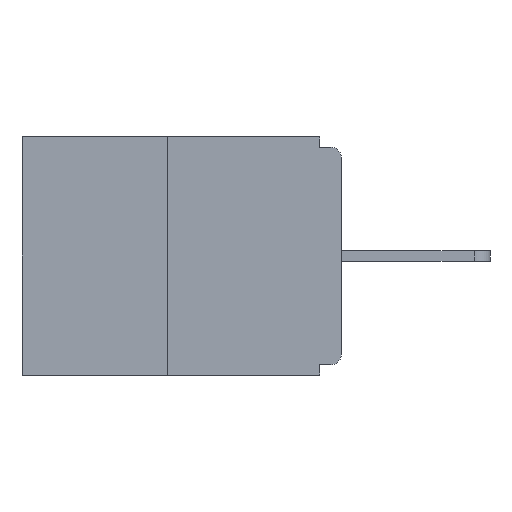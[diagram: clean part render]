
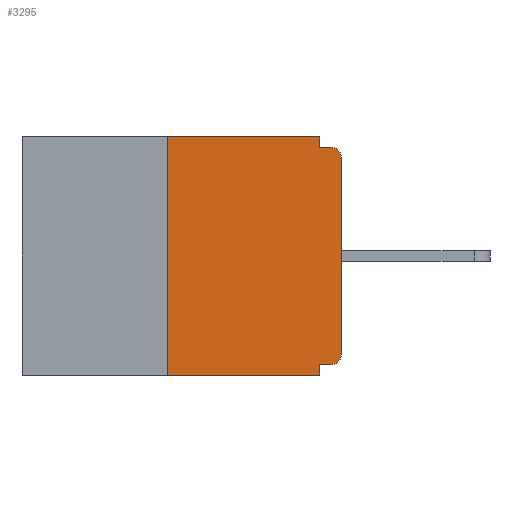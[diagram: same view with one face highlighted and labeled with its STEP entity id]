
A CAD part, left-side view. The second image highlights one B-rep face of the part: STEP entity #3295.
In plain terms, the highlighted planar face has unit normal (-1, 0, 0).
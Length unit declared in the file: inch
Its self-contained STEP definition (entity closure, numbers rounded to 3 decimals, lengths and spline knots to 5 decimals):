
#161 = VECTOR ( 'NONE', #1043, 39.37008 ) ;
#239 = DIRECTION ( 'NONE',  ( 0., 0., -1. ) ) ;
#423 = EDGE_CURVE ( 'NONE', #15129, #9953, #10699, .T. ) ;
#1043 = DIRECTION ( 'NONE',  ( 0., 0., -1. ) ) ;
#1128 = VERTEX_POINT ( 'NONE', #9531 ) ;
#1290 = VECTOR ( 'NONE', #1353, 39.37008 ) ;
#1353 = DIRECTION ( 'NONE',  ( 0., -1., 0. ) ) ;
#1645 = LINE ( 'NONE', #8668, #11271 ) ;
#2139 = EDGE_CURVE ( 'NONE', #6346, #11528, #9240, .T. ) ;
#2276 = ORIENTED_EDGE ( 'NONE', *, *, #6150, .F. ) ;
#3017 = EDGE_CURVE ( 'NONE', #9953, #8100, #14920, .T. ) ;
#3056 = CARTESIAN_POINT ( 'NONE',  ( 0., 0.015, -0.328 ) ) ;
#3295 = ADVANCED_FACE ( 'NONE', ( #3906 ), #15414, .F. ) ;
#3436 = VECTOR ( 'NONE', #5812, 39.37008 ) ;
#3559 = ORIENTED_EDGE ( 'NONE', *, *, #3017, .F. ) ;
#3906 = FACE_OUTER_BOUND ( 'NONE', #9827, .T. ) ;
#4535 = VECTOR ( 'NONE', #5402, 39.37008 ) ;
#4733 = EDGE_CURVE ( 'NONE', #5735, #5807, #5259, .T. ) ;
#4898 = DIRECTION ( 'NONE',  ( -1., 0., 0. ) ) ;
#5259 = LINE ( 'NONE', #17014, #1290 ) ;
#5402 = DIRECTION ( 'NONE',  ( 0., -1., 0. ) ) ;
#5409 = AXIS2_PLACEMENT_3D ( 'NONE', #15993, #8215, #239 ) ;
#5502 = CARTESIAN_POINT ( 'NONE',  ( 0., 0., -0.015 ) ) ;
#5602 = CARTESIAN_POINT ( 'NONE',  ( 0., 0.031, 0. ) ) ;
#5735 = VERTEX_POINT ( 'NONE', #14132 ) ;
#5807 = VERTEX_POINT ( 'NONE', #12951 ) ;
#5812 = DIRECTION ( 'NONE',  ( 0., 0., -1. ) ) ;
#5891 = DIRECTION ( 'NONE',  ( 0., 0., 1. ) ) ;
#6026 = VECTOR ( 'NONE', #13220, 39.37008 ) ;
#6150 = EDGE_CURVE ( 'NONE', #7474, #5807, #13802, .T. ) ;
#6218 = VECTOR ( 'NONE', #5891, 39.37008 ) ;
#6346 = VERTEX_POINT ( 'NONE', #12648 ) ;
#7019 = ORIENTED_EDGE ( 'NONE', *, *, #423, .F. ) ;
#7474 = VERTEX_POINT ( 'NONE', #14976 ) ;
#7567 = EDGE_CURVE ( 'NONE', #5735, #1128, #1645, .T. ) ;
#7932 = EDGE_CURVE ( 'NONE', #1128, #15129, #9456, .T. ) ;
#8100 = VERTEX_POINT ( 'NONE', #14905 ) ;
#8114 = AXIS2_PLACEMENT_3D ( 'NONE', #15377, #15322, #15286 ) ;
#8215 = DIRECTION ( 'NONE',  ( -1., 0., 0. ) ) ;
#8668 = CARTESIAN_POINT ( 'NONE',  ( 0., 0.25, 0. ) ) ;
#9099 = VECTOR ( 'NONE', #14774, 39.37008 ) ;
#9237 = ORIENTED_EDGE ( 'NONE', *, *, #15153, .F. ) ;
#9240 = LINE ( 'NONE', #12000, #6218 ) ;
#9430 = EDGE_CURVE ( 'NONE', #11528, #8100, #13034, .T. ) ;
#9456 = LINE ( 'NONE', #11881, #6026 ) ;
#9525 = CARTESIAN_POINT ( 'NONE',  ( 0., 0., -0.328 ) ) ;
#9531 = CARTESIAN_POINT ( 'NONE',  ( 0., 0.25, 0. ) ) ;
#9643 = ORIENTED_EDGE ( 'NONE', *, *, #2139, .T. ) ;
#9725 = CARTESIAN_POINT ( 'NONE',  ( 0., 0.031, -0.343 ) ) ;
#9827 = EDGE_LOOP ( 'NONE', ( #11824, #12253, #15743, #2276, #9237, #12660, #9643, #13074, #3559, #7019 ) ) ;
#9945 = DIRECTION ( 'NONE',  ( 0., 0., 1. ) ) ;
#9953 = VERTEX_POINT ( 'NONE', #12525 ) ;
#10699 = LINE ( 'NONE', #12511, #161 ) ;
#11271 = VECTOR ( 'NONE', #9945, 39.37008 ) ;
#11528 = VERTEX_POINT ( 'NONE', #14765 ) ;
#11824 = ORIENTED_EDGE ( 'NONE', *, *, #7932, .F. ) ;
#11881 = CARTESIAN_POINT ( 'NONE',  ( 0., 0.46, 0. ) ) ;
#12000 = CARTESIAN_POINT ( 'NONE',  ( 0., 0., 0. ) ) ;
#12253 = ORIENTED_EDGE ( 'NONE', *, *, #7567, .F. ) ;
#12511 = CARTESIAN_POINT ( 'NONE',  ( 0., 0.031, 0. ) ) ;
#12525 = CARTESIAN_POINT ( 'NONE',  ( 0., 0.031, -0.015 ) ) ;
#12648 = CARTESIAN_POINT ( 'NONE',  ( 0., 0., -0.313 ) ) ;
#12653 = CARTESIAN_POINT ( 'NONE',  ( 0., 0.015, -0.03 ) ) ;
#12660 = ORIENTED_EDGE ( 'NONE', *, *, #15756, .T. ) ;
#12951 = CARTESIAN_POINT ( 'NONE',  ( 0., 0.031, -0.343 ) ) ;
#13034 = CIRCLE ( 'NONE', #15487, 0.015 ) ;
#13074 = ORIENTED_EDGE ( 'NONE', *, *, #9430, .T. ) ;
#13220 = DIRECTION ( 'NONE',  ( 0., -1., 0. ) ) ;
#13802 = LINE ( 'NONE', #9725, #3436 ) ;
#13962 = CIRCLE ( 'NONE', #5409, 0.015 ) ;
#14002 = DIRECTION ( 'NONE',  ( 0., 0., -1. ) ) ;
#14132 = CARTESIAN_POINT ( 'NONE',  ( 0., 0.25, -0.343 ) ) ;
#14555 = VERTEX_POINT ( 'NONE', #3056 ) ;
#14765 = CARTESIAN_POINT ( 'NONE',  ( 0., 0., -0.03 ) ) ;
#14774 = DIRECTION ( 'NONE',  ( 0., 1., 0. ) ) ;
#14905 = CARTESIAN_POINT ( 'NONE',  ( 0., 0.015, -0.015 ) ) ;
#14920 = LINE ( 'NONE', #5502, #4535 ) ;
#14976 = CARTESIAN_POINT ( 'NONE',  ( 0., 0.031, -0.328 ) ) ;
#15129 = VERTEX_POINT ( 'NONE', #5602 ) ;
#15153 = EDGE_CURVE ( 'NONE', #14555, #7474, #16004, .T. ) ;
#15286 = DIRECTION ( 'NONE',  ( 0., 0., -1. ) ) ;
#15322 = DIRECTION ( 'NONE',  ( 1., 0., 0. ) ) ;
#15377 = CARTESIAN_POINT ( 'NONE',  ( 0., 0.46, 0. ) ) ;
#15414 = PLANE ( 'NONE',  #8114 ) ;
#15487 = AXIS2_PLACEMENT_3D ( 'NONE', #12653, #4898, #14002 ) ;
#15743 = ORIENTED_EDGE ( 'NONE', *, *, #4733, .T. ) ;
#15756 = EDGE_CURVE ( 'NONE', #14555, #6346, #13962, .T. ) ;
#15993 = CARTESIAN_POINT ( 'NONE',  ( 0., 0.015, -0.313 ) ) ;
#16004 = LINE ( 'NONE', #9525, #9099 ) ;
#17014 = CARTESIAN_POINT ( 'NONE',  ( 0., 0.46, -0.343 ) ) ;
